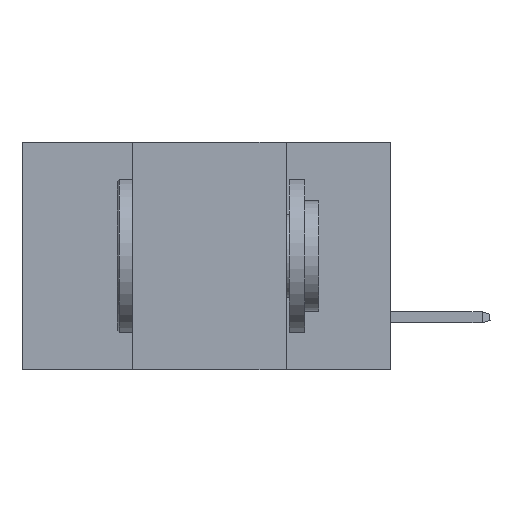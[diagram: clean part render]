
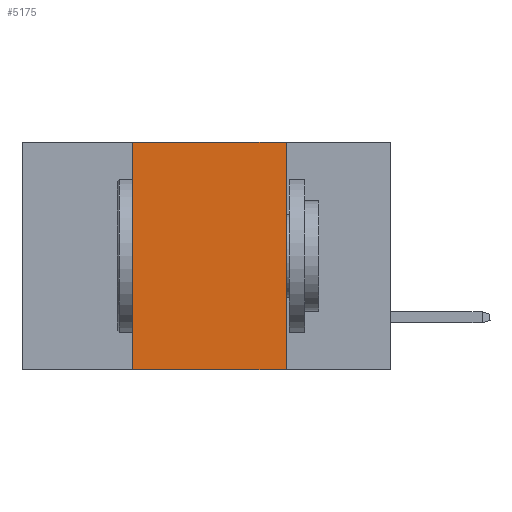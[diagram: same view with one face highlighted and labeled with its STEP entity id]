
A CAD part, left-side view. The second image highlights one B-rep face of the part: STEP entity #5175.
In plain terms, the highlighted planar face has unit normal (-1, 0, 0).
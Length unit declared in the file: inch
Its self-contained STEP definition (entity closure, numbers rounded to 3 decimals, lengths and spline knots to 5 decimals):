
#1208 = VERTEX_POINT ( 'NONE', #3612 ) ;
#3491 = VERTEX_POINT ( 'NONE', #9739 ) ;
#3612 = CARTESIAN_POINT ( 'NONE',  ( 0., 0.42, 0. ) ) ;
#5175 = ADVANCED_FACE ( 'NONE', ( #17752 ), #7897, .F. ) ;
#7625 = EDGE_CURVE ( 'NONE', #1208, #20606, #29218, .T. ) ;
#7877 = CARTESIAN_POINT ( 'NONE',  ( 0., 0.6, 0. ) ) ;
#7897 = PLANE ( 'NONE',  #30203 ) ;
#7948 = ORIENTED_EDGE ( 'NONE', *, *, #7625, .F. ) ;
#8290 = LINE ( 'NONE', #14352, #29087 ) ;
#9429 = EDGE_CURVE ( 'NONE', #22131, #1208, #8290, .T. ) ;
#9739 = CARTESIAN_POINT ( 'NONE',  ( 0., 0.17, -0.37 ) ) ;
#10375 = CARTESIAN_POINT ( 'NONE',  ( 0., 0.17, 0. ) ) ;
#11564 = CARTESIAN_POINT ( 'NONE',  ( 0., 0.6, -0.37 ) ) ;
#12141 = ORIENTED_EDGE ( 'NONE', *, *, #9429, .F. ) ;
#12536 = CARTESIAN_POINT ( 'NONE',  ( 0., 0.6, 0. ) ) ;
#12840 = DIRECTION ( 'NONE',  ( 1., 0., 0. ) ) ;
#13533 = ORIENTED_EDGE ( 'NONE', *, *, #28248, .T. ) ;
#13584 = EDGE_LOOP ( 'NONE', ( #17654, #7948, #12141, #13533 ) ) ;
#14352 = CARTESIAN_POINT ( 'NONE',  ( 0., 0.42, 0. ) ) ;
#15327 = DIRECTION ( 'NONE',  ( 0., 0., -1. ) ) ;
#15373 = DIRECTION ( 'NONE',  ( 0., 0., -1. ) ) ;
#17654 = ORIENTED_EDGE ( 'NONE', *, *, #26097, .F. ) ;
#17752 = FACE_OUTER_BOUND ( 'NONE', #13584, .T. ) ;
#17866 = CARTESIAN_POINT ( 'NONE',  ( 0., 0.17, 0. ) ) ;
#19496 = CARTESIAN_POINT ( 'NONE',  ( 0., 0.42, -0.37 ) ) ;
#20581 = LINE ( 'NONE', #11564, #30751 ) ;
#20606 = VERTEX_POINT ( 'NONE', #17866 ) ;
#22131 = VERTEX_POINT ( 'NONE', #19496 ) ;
#22278 = DIRECTION ( 'NONE',  ( 0., 0., 1. ) ) ;
#25877 = VECTOR ( 'NONE', #15373, 39.37008 ) ;
#26097 = EDGE_CURVE ( 'NONE', #20606, #3491, #26290, .T. ) ;
#26290 = LINE ( 'NONE', #10375, #25877 ) ;
#26590 = DIRECTION ( 'NONE',  ( 0., -1., 0. ) ) ;
#28248 = EDGE_CURVE ( 'NONE', #22131, #3491, #20581, .T. ) ;
#28375 = VECTOR ( 'NONE', #30418, 39.37008 ) ;
#29087 = VECTOR ( 'NONE', #22278, 39.37008 ) ;
#29218 = LINE ( 'NONE', #7877, #28375 ) ;
#30203 = AXIS2_PLACEMENT_3D ( 'NONE', #12536, #12840, #15327 ) ;
#30418 = DIRECTION ( 'NONE',  ( 0., -1., 0. ) ) ;
#30751 = VECTOR ( 'NONE', #26590, 39.37008 ) ;
